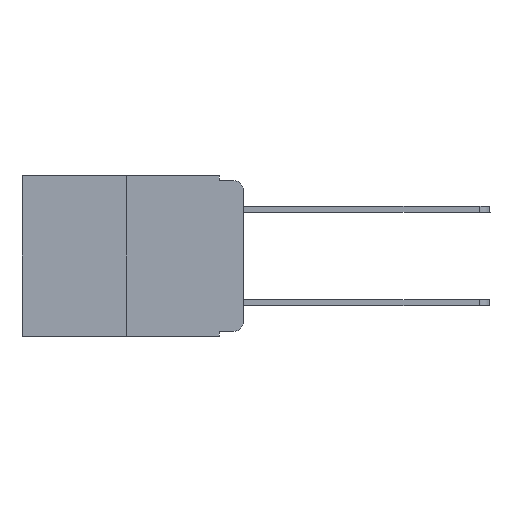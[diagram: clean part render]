
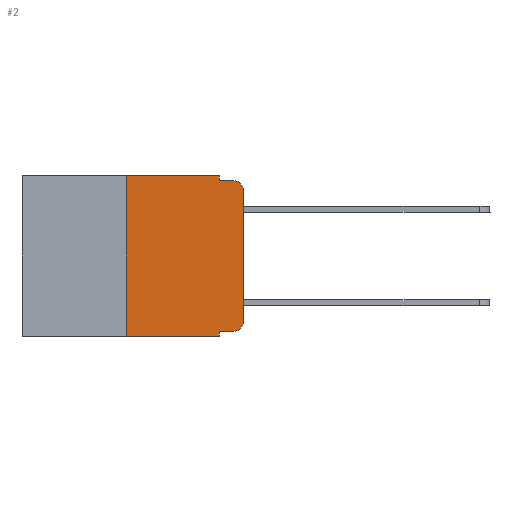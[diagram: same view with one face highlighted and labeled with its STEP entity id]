
A CAD part, left-side view. The second image highlights one B-rep face of the part: STEP entity #2.
In plain terms, the highlighted planar face has unit normal (-1, 0, 0).
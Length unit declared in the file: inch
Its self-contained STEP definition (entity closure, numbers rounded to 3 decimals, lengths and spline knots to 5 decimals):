
#2 = ADVANCED_FACE ( 'NONE', ( #24297 ), #7946, .F. ) ;
#16 = VERTEX_POINT ( 'NONE', #24539 ) ;
#1104 = EDGE_CURVE ( 'NONE', #13208, #11058, #17778, .T. ) ;
#1124 = ORIENTED_EDGE ( 'NONE', *, *, #17679, .T. ) ;
#1247 = DIRECTION ( 'NONE',  ( 0., 0., -1. ) ) ;
#1851 = CIRCLE ( 'NONE', #24591, 0.02 ) ;
#2256 = VERTEX_POINT ( 'NONE', #18873 ) ;
#2427 = CARTESIAN_POINT ( 'NONE',  ( 0., 0.02, -0.333 ) ) ;
#2759 = DIRECTION ( 'NONE',  ( 0., 0., 1. ) ) ;
#2767 = EDGE_CURVE ( 'NONE', #4194, #21774, #1851, .T. ) ;
#3704 = CARTESIAN_POINT ( 'NONE',  ( 0., 0.25, -0.343 ) ) ;
#3991 = ORIENTED_EDGE ( 'NONE', *, *, #1104, .F. ) ;
#4002 = AXIS2_PLACEMENT_3D ( 'NONE', #7132, #6782, #12995 ) ;
#4194 = VERTEX_POINT ( 'NONE', #19701 ) ;
#4221 = DIRECTION ( 'NONE',  ( 0., -1., 0. ) ) ;
#4435 = DIRECTION ( 'NONE',  ( 0., -1., 0. ) ) ;
#4642 = EDGE_CURVE ( 'NONE', #2256, #8457, #22061, .T. ) ;
#4910 = ORIENTED_EDGE ( 'NONE', *, *, #2767, .T. ) ;
#5072 = EDGE_CURVE ( 'NONE', #11058, #2256, #19609, .T. ) ;
#5204 = EDGE_CURVE ( 'NONE', #16555, #16, #11280, .T. ) ;
#5753 = ORIENTED_EDGE ( 'NONE', *, *, #5204, .F. ) ;
#6244 = CARTESIAN_POINT ( 'NONE',  ( 0., 0.473, 0. ) ) ;
#6273 = CARTESIAN_POINT ( 'NONE',  ( 0., 0.473, -0.343 ) ) ;
#6558 = VERTEX_POINT ( 'NONE', #15858 ) ;
#6691 = LINE ( 'NONE', #6273, #24583 ) ;
#6782 = DIRECTION ( 'NONE',  ( -1., 0., 0. ) ) ;
#7037 = ORIENTED_EDGE ( 'NONE', *, *, #10420, .T. ) ;
#7132 = CARTESIAN_POINT ( 'NONE',  ( 0., 0.02, -0.313 ) ) ;
#7514 = VECTOR ( 'NONE', #13728, 39.37008 ) ;
#7630 = CARTESIAN_POINT ( 'NONE',  ( 0., 0.02, -0.01 ) ) ;
#7930 = CIRCLE ( 'NONE', #4002, 0.02 ) ;
#7946 = PLANE ( 'NONE',  #21085 ) ;
#8012 = ORIENTED_EDGE ( 'NONE', *, *, #13483, .T. ) ;
#8457 = VERTEX_POINT ( 'NONE', #16907 ) ;
#8658 = CARTESIAN_POINT ( 'NONE',  ( 0., 0.051, -0.333 ) ) ;
#9610 = DIRECTION ( 'NONE',  ( 0., 0., 1. ) ) ;
#9779 = CARTESIAN_POINT ( 'NONE',  ( 0., 0.051, -0.333 ) ) ;
#10262 = CARTESIAN_POINT ( 'NONE',  ( 0., 0.473, 0. ) ) ;
#10420 = EDGE_CURVE ( 'NONE', #13208, #16, #6691, .T. ) ;
#10528 = ORIENTED_EDGE ( 'NONE', *, *, #5072, .F. ) ;
#10796 = VECTOR ( 'NONE', #9610, 39.37008 ) ;
#11058 = VERTEX_POINT ( 'NONE', #12789 ) ;
#11280 = LINE ( 'NONE', #14322, #15587 ) ;
#12553 = VECTOR ( 'NONE', #2759, 39.37008 ) ;
#12596 = CARTESIAN_POINT ( 'NONE',  ( 0., 0.25, 0. ) ) ;
#12789 = CARTESIAN_POINT ( 'NONE',  ( 0., 0.25, 0. ) ) ;
#12968 = VERTEX_POINT ( 'NONE', #2427 ) ;
#12995 = DIRECTION ( 'NONE',  ( 0., 0., -1. ) ) ;
#13208 = VERTEX_POINT ( 'NONE', #3704 ) ;
#13483 = EDGE_CURVE ( 'NONE', #16555, #12968, #18893, .T. ) ;
#13556 = CARTESIAN_POINT ( 'NONE',  ( 0., 0.02, -0.03 ) ) ;
#13647 = ORIENTED_EDGE ( 'NONE', *, *, #4642, .F. ) ;
#13728 = DIRECTION ( 'NONE',  ( 0., -1., 0. ) ) ;
#14322 = CARTESIAN_POINT ( 'NONE',  ( 0., 0.051, 0. ) ) ;
#14610 = CARTESIAN_POINT ( 'NONE',  ( 0., 0.051, -0.01 ) ) ;
#15587 = VECTOR ( 'NONE', #20439, 39.37008 ) ;
#15858 = CARTESIAN_POINT ( 'NONE',  ( 0., 0., -0.313 ) ) ;
#16098 = ORIENTED_EDGE ( 'NONE', *, *, #20538, .F. ) ;
#16555 = VERTEX_POINT ( 'NONE', #8658 ) ;
#16907 = CARTESIAN_POINT ( 'NONE',  ( 0., 0.051, -0.01 ) ) ;
#17172 = DIRECTION ( 'NONE',  ( 0., 0., -1. ) ) ;
#17411 = ORIENTED_EDGE ( 'NONE', *, *, #22253, .T. ) ;
#17679 = EDGE_CURVE ( 'NONE', #12968, #6558, #7930, .T. ) ;
#17778 = LINE ( 'NONE', #12596, #12553 ) ;
#18686 = VECTOR ( 'NONE', #1247, 39.37008 ) ;
#18873 = CARTESIAN_POINT ( 'NONE',  ( 0., 0.051, 0. ) ) ;
#18893 = LINE ( 'NONE', #9779, #20431 ) ;
#19034 = DIRECTION ( 'NONE',  ( 0., 0., -1. ) ) ;
#19609 = LINE ( 'NONE', #6244, #20519 ) ;
#19701 = CARTESIAN_POINT ( 'NONE',  ( 0., 0., -0.03 ) ) ;
#20431 = VECTOR ( 'NONE', #4221, 39.37008 ) ;
#20439 = DIRECTION ( 'NONE',  ( 0., 0., -1. ) ) ;
#20519 = VECTOR ( 'NONE', #24057, 39.37008 ) ;
#20538 = EDGE_CURVE ( 'NONE', #8457, #21774, #24760, .T. ) ;
#21085 = AXIS2_PLACEMENT_3D ( 'NONE', #10262, #22470, #19034 ) ;
#21140 = CARTESIAN_POINT ( 'NONE',  ( 0., 0.051, 0. ) ) ;
#21294 = DIRECTION ( 'NONE',  ( -1., 0., 0. ) ) ;
#21426 = EDGE_LOOP ( 'NONE', ( #17411, #4910, #16098, #13647, #10528, #3991, #7037, #5753, #8012, #1124 ) ) ;
#21774 = VERTEX_POINT ( 'NONE', #7630 ) ;
#22061 = LINE ( 'NONE', #21140, #18686 ) ;
#22253 = EDGE_CURVE ( 'NONE', #6558, #4194, #23738, .T. ) ;
#22470 = DIRECTION ( 'NONE',  ( 1., 0., 0. ) ) ;
#23738 = LINE ( 'NONE', #25385, #10796 ) ;
#24057 = DIRECTION ( 'NONE',  ( 0., -1., 0. ) ) ;
#24297 = FACE_OUTER_BOUND ( 'NONE', #21426, .T. ) ;
#24539 = CARTESIAN_POINT ( 'NONE',  ( 0., 0.051, -0.343 ) ) ;
#24583 = VECTOR ( 'NONE', #4435, 39.37008 ) ;
#24591 = AXIS2_PLACEMENT_3D ( 'NONE', #13556, #21294, #17172 ) ;
#24760 = LINE ( 'NONE', #14610, #7514 ) ;
#25385 = CARTESIAN_POINT ( 'NONE',  ( 0., 0., 0. ) ) ;
